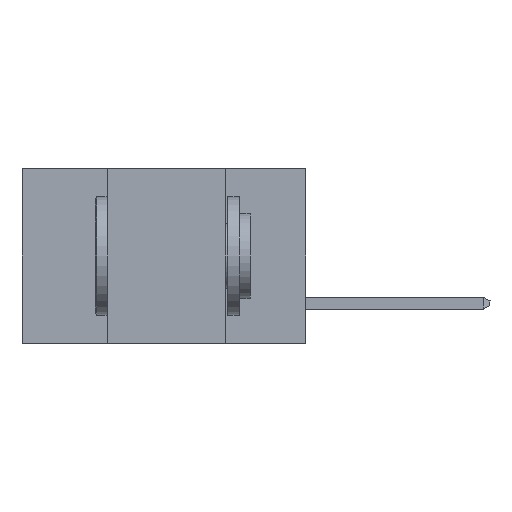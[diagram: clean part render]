
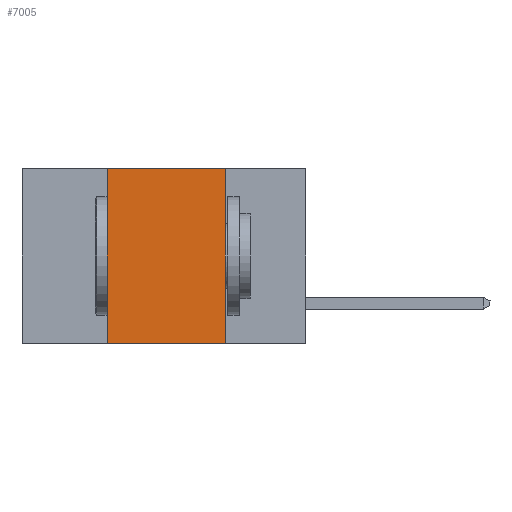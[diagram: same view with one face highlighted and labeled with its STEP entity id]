
A CAD part, left-side view. The second image highlights one B-rep face of the part: STEP entity #7005.
In plain terms, the highlighted planar face has unit normal (-1, 0, 0).
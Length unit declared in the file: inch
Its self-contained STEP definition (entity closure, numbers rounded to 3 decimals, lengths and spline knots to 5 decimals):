
#1497 = DIRECTION ( 'NONE',  ( 0., 0., 1. ) ) ;
#2110 = FACE_OUTER_BOUND ( 'NONE', #13207, .T. ) ;
#2336 = LINE ( 'NONE', #9466, #9776 ) ;
#3208 = DIRECTION ( 'NONE',  ( 1., 0., 0. ) ) ;
#3251 = CARTESIAN_POINT ( 'NONE',  ( 0., 0.17, -0.37 ) ) ;
#3264 = EDGE_CURVE ( 'NONE', #16027, #13792, #17741, .T. ) ;
#3465 = CARTESIAN_POINT ( 'NONE',  ( 0., 0.6, 0. ) ) ;
#3501 = ORIENTED_EDGE ( 'NONE', *, *, #3264, .F. ) ;
#4346 = ORIENTED_EDGE ( 'NONE', *, *, #15425, .F. ) ;
#4552 = DIRECTION ( 'NONE',  ( 0., -1., 0. ) ) ;
#4724 = VECTOR ( 'NONE', #15114, 39.37008 ) ;
#5359 = AXIS2_PLACEMENT_3D ( 'NONE', #10407, #3208, #15112 ) ;
#6181 = CARTESIAN_POINT ( 'NONE',  ( 0., 0.6, -0.37 ) ) ;
#6539 = ORIENTED_EDGE ( 'NONE', *, *, #10901, .T. ) ;
#7005 = ADVANCED_FACE ( 'NONE', ( #2110 ), #13564, .F. ) ;
#8007 = CARTESIAN_POINT ( 'NONE',  ( 0., 0.42, -0.37 ) ) ;
#8339 = ORIENTED_EDGE ( 'NONE', *, *, #16632, .F. ) ;
#8669 = LINE ( 'NONE', #3465, #4724 ) ;
#9466 = CARTESIAN_POINT ( 'NONE',  ( 0., 0.17, 0. ) ) ;
#9511 = CARTESIAN_POINT ( 'NONE',  ( 0., 0.42, 0. ) ) ;
#9772 = VERTEX_POINT ( 'NONE', #3251 ) ;
#9776 = VECTOR ( 'NONE', #15259, 39.37008 ) ;
#10407 = CARTESIAN_POINT ( 'NONE',  ( 0., 0.6, 0. ) ) ;
#10901 = EDGE_CURVE ( 'NONE', #16027, #9772, #18404, .T. ) ;
#12737 = CARTESIAN_POINT ( 'NONE',  ( 0., 0.17, 0. ) ) ;
#13207 = EDGE_LOOP ( 'NONE', ( #8339, #4346, #3501, #6539 ) ) ;
#13516 = VERTEX_POINT ( 'NONE', #12737 ) ;
#13564 = PLANE ( 'NONE',  #5359 ) ;
#13792 = VERTEX_POINT ( 'NONE', #9511 ) ;
#15112 = DIRECTION ( 'NONE',  ( 0., 0., -1. ) ) ;
#15114 = DIRECTION ( 'NONE',  ( 0., -1., 0. ) ) ;
#15259 = DIRECTION ( 'NONE',  ( 0., 0., -1. ) ) ;
#15396 = VECTOR ( 'NONE', #4552, 39.37008 ) ;
#15425 = EDGE_CURVE ( 'NONE', #13792, #13516, #8669, .T. ) ;
#16027 = VERTEX_POINT ( 'NONE', #8007 ) ;
#16211 = CARTESIAN_POINT ( 'NONE',  ( 0., 0.42, 0. ) ) ;
#16632 = EDGE_CURVE ( 'NONE', #13516, #9772, #2336, .T. ) ;
#16791 = VECTOR ( 'NONE', #1497, 39.37008 ) ;
#17741 = LINE ( 'NONE', #16211, #16791 ) ;
#18404 = LINE ( 'NONE', #6181, #15396 ) ;
